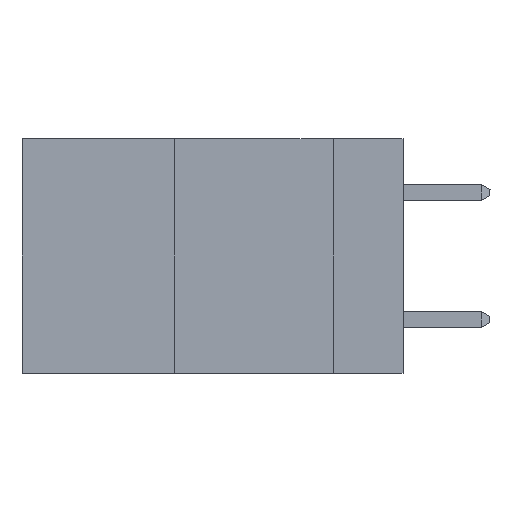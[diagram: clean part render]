
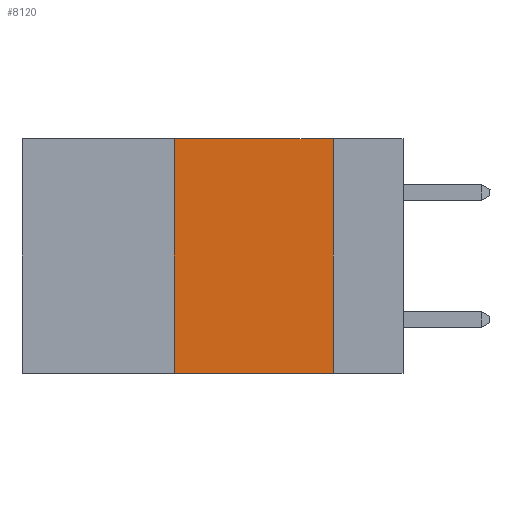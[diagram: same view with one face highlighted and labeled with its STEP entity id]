
A CAD part, left-side view. The second image highlights one B-rep face of the part: STEP entity #8120.
In plain terms, the highlighted planar face has unit normal (-1, 0, 0).
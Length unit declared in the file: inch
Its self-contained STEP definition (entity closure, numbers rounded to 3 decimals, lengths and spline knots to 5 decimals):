
#771 = ORIENTED_EDGE ( 'NONE', *, *, #2596, .T. ) ;
#1913 = DIRECTION ( 'NONE',  ( 0., -1., 0. ) ) ;
#2596 = EDGE_CURVE ( 'NONE', #11422, #20917, #7769, .T. ) ;
#4574 = LINE ( 'NONE', #13641, #5209 ) ;
#5209 = VECTOR ( 'NONE', #1913, 39.37008 ) ;
#5677 = LINE ( 'NONE', #10484, #10248 ) ;
#7496 = DIRECTION ( 'NONE',  ( 0., 0., -1. ) ) ;
#7769 = LINE ( 'NONE', #13694, #10185 ) ;
#8120 = ADVANCED_FACE ( 'NONE', ( #18550 ), #23704, .F. ) ;
#9349 = EDGE_LOOP ( 'NONE', ( #24504, #10440, #15647, #771 ) ) ;
#10185 = VECTOR ( 'NONE', #19653, 39.37008 ) ;
#10248 = VECTOR ( 'NONE', #16232, 39.37008 ) ;
#10440 = ORIENTED_EDGE ( 'NONE', *, *, #15625, .F. ) ;
#10484 = CARTESIAN_POINT ( 'NONE',  ( 0., 0.36, 0. ) ) ;
#11422 = VERTEX_POINT ( 'NONE', #24098 ) ;
#12684 = EDGE_CURVE ( 'NONE', #11422, #15314, #5677, .T. ) ;
#13641 = CARTESIAN_POINT ( 'NONE',  ( 0., 0.6, 0. ) ) ;
#13694 = CARTESIAN_POINT ( 'NONE',  ( 0., 0.6, -0.37 ) ) ;
#14061 = VECTOR ( 'NONE', #7496, 39.37008 ) ;
#15314 = VERTEX_POINT ( 'NONE', #24595 ) ;
#15625 = EDGE_CURVE ( 'NONE', #15314, #21587, #4574, .T. ) ;
#15647 = ORIENTED_EDGE ( 'NONE', *, *, #12684, .F. ) ;
#16130 = EDGE_CURVE ( 'NONE', #21587, #20917, #25053, .T. ) ;
#16232 = DIRECTION ( 'NONE',  ( 0., 0., 1. ) ) ;
#18111 = CARTESIAN_POINT ( 'NONE',  ( 0., 0.6, 0. ) ) ;
#18550 = FACE_OUTER_BOUND ( 'NONE', #9349, .T. ) ;
#18598 = AXIS2_PLACEMENT_3D ( 'NONE', #18111, #24203, #21992 ) ;
#19239 = CARTESIAN_POINT ( 'NONE',  ( 0., 0.11, 0. ) ) ;
#19653 = DIRECTION ( 'NONE',  ( 0., -1., 0. ) ) ;
#20917 = VERTEX_POINT ( 'NONE', #24976 ) ;
#21054 = CARTESIAN_POINT ( 'NONE',  ( 0., 0.11, 0. ) ) ;
#21587 = VERTEX_POINT ( 'NONE', #21054 ) ;
#21992 = DIRECTION ( 'NONE',  ( 0., 0., -1. ) ) ;
#23704 = PLANE ( 'NONE',  #18598 ) ;
#24098 = CARTESIAN_POINT ( 'NONE',  ( 0., 0.36, -0.37 ) ) ;
#24203 = DIRECTION ( 'NONE',  ( 1., 0., 0. ) ) ;
#24504 = ORIENTED_EDGE ( 'NONE', *, *, #16130, .F. ) ;
#24595 = CARTESIAN_POINT ( 'NONE',  ( 0., 0.36, 0. ) ) ;
#24976 = CARTESIAN_POINT ( 'NONE',  ( 0., 0.11, -0.37 ) ) ;
#25053 = LINE ( 'NONE', #19239, #14061 ) ;
